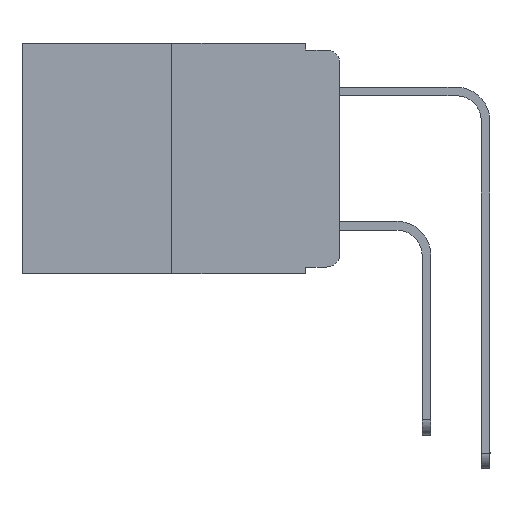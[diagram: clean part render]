
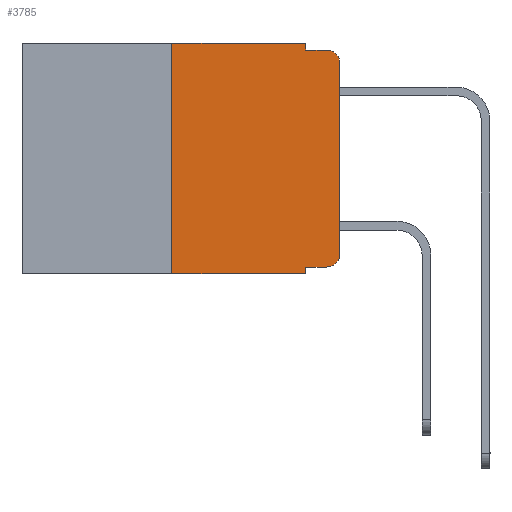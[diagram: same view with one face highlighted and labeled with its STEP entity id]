
A CAD part, left-side view. The second image highlights one B-rep face of the part: STEP entity #3785.
In plain terms, the highlighted planar face has unit normal (-1, 0, 0).
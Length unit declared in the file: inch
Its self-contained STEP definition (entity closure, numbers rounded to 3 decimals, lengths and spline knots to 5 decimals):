
#272 = LINE ( 'NONE', #19175, #15373 ) ;
#403 = CARTESIAN_POINT ( 'NONE',  ( 0., 0.25, 0. ) ) ;
#550 = VECTOR ( 'NONE', #16268, 39.37008 ) ;
#668 = VERTEX_POINT ( 'NONE', #17638 ) ;
#694 = CARTESIAN_POINT ( 'NONE',  ( 0., 0.051, -0.01 ) ) ;
#1282 = DIRECTION ( 'NONE',  ( 0., -1., 0. ) ) ;
#1435 = ORIENTED_EDGE ( 'NONE', *, *, #10564, .T. ) ;
#1475 = VERTEX_POINT ( 'NONE', #15623 ) ;
#1522 = DIRECTION ( 'NONE',  ( 0., -1., 0. ) ) ;
#1598 = CARTESIAN_POINT ( 'NONE',  ( 0., 0.02, -0.03 ) ) ;
#1801 = ORIENTED_EDGE ( 'NONE', *, *, #5862, .F. ) ;
#2607 = EDGE_CURVE ( 'NONE', #5838, #4358, #6332, .T. ) ;
#2641 = VERTEX_POINT ( 'NONE', #694 ) ;
#2734 = DIRECTION ( 'NONE',  ( 1., 0., 0. ) ) ;
#2908 = CIRCLE ( 'NONE', #12772, 0.02 ) ;
#3041 = ORIENTED_EDGE ( 'NONE', *, *, #8860, .F. ) ;
#3785 = ADVANCED_FACE ( 'NONE', ( #19972 ), #5840, .F. ) ;
#4199 = EDGE_CURVE ( 'NONE', #2641, #15779, #15564, .T. ) ;
#4358 = VERTEX_POINT ( 'NONE', #5074 ) ;
#4438 = VERTEX_POINT ( 'NONE', #11540 ) ;
#4927 = CIRCLE ( 'NONE', #16407, 0.02 ) ;
#5074 = CARTESIAN_POINT ( 'NONE',  ( 0., 0.051, 0. ) ) ;
#5301 = CARTESIAN_POINT ( 'NONE',  ( 0., 0.051, 0. ) ) ;
#5365 = LINE ( 'NONE', #9783, #550 ) ;
#5838 = VERTEX_POINT ( 'NONE', #15983 ) ;
#5839 = VERTEX_POINT ( 'NONE', #11443 ) ;
#5840 = PLANE ( 'NONE',  #17821 ) ;
#5862 = EDGE_CURVE ( 'NONE', #20322, #5838, #8253, .T. ) ;
#6332 = LINE ( 'NONE', #6436, #11780 ) ;
#6436 = CARTESIAN_POINT ( 'NONE',  ( 0., 0.473, 0. ) ) ;
#6742 = DIRECTION ( 'NONE',  ( -1., 0., 0. ) ) ;
#7667 = EDGE_LOOP ( 'NONE', ( #11766, #1435, #14814, #20324, #12751, #1801, #14634, #3041, #14861, #11894 ) ) ;
#7842 = DIRECTION ( 'NONE',  ( 0., -1., 0. ) ) ;
#8253 = LINE ( 'NONE', #403, #8597 ) ;
#8597 = VECTOR ( 'NONE', #11545, 39.37008 ) ;
#8860 = EDGE_CURVE ( 'NONE', #1475, #4438, #19435, .T. ) ;
#9343 = CARTESIAN_POINT ( 'NONE',  ( 0., 0.473, -0.343 ) ) ;
#9572 = CARTESIAN_POINT ( 'NONE',  ( 0., 0.25, -0.343 ) ) ;
#9783 = CARTESIAN_POINT ( 'NONE',  ( 0., 0., 0. ) ) ;
#10564 = EDGE_CURVE ( 'NONE', #668, #15779, #2908, .T. ) ;
#10661 = EDGE_CURVE ( 'NONE', #18608, #5839, #4927, .T. ) ;
#11046 = CARTESIAN_POINT ( 'NONE',  ( 0., 0.02, -0.01 ) ) ;
#11156 = VECTOR ( 'NONE', #14761, 39.37008 ) ;
#11443 = CARTESIAN_POINT ( 'NONE',  ( 0., 0., -0.313 ) ) ;
#11540 = CARTESIAN_POINT ( 'NONE',  ( 0., 0.051, -0.343 ) ) ;
#11545 = DIRECTION ( 'NONE',  ( 0., 0., 1. ) ) ;
#11766 = ORIENTED_EDGE ( 'NONE', *, *, #17537, .T. ) ;
#11780 = VECTOR ( 'NONE', #1282, 39.37008 ) ;
#11827 = EDGE_CURVE ( 'NONE', #20322, #4438, #12431, .T. ) ;
#11894 = ORIENTED_EDGE ( 'NONE', *, *, #10661, .T. ) ;
#12172 = CARTESIAN_POINT ( 'NONE',  ( 0., 0.051, -0.333 ) ) ;
#12431 = LINE ( 'NONE', #9343, #12601 ) ;
#12601 = VECTOR ( 'NONE', #1522, 39.37008 ) ;
#12751 = ORIENTED_EDGE ( 'NONE', *, *, #2607, .F. ) ;
#12772 = AXIS2_PLACEMENT_3D ( 'NONE', #1598, #6742, #14370 ) ;
#12940 = VECTOR ( 'NONE', #7842, 39.37008 ) ;
#13179 = CARTESIAN_POINT ( 'NONE',  ( 0., 0.02, -0.333 ) ) ;
#13204 = CARTESIAN_POINT ( 'NONE',  ( 0., 0.02, -0.313 ) ) ;
#13825 = DIRECTION ( 'NONE',  ( 0., -1., 0. ) ) ;
#14370 = DIRECTION ( 'NONE',  ( 0., 0., -1. ) ) ;
#14634 = ORIENTED_EDGE ( 'NONE', *, *, #11827, .T. ) ;
#14675 = DIRECTION ( 'NONE',  ( 0., 0., -1. ) ) ;
#14761 = DIRECTION ( 'NONE',  ( 0., 0., -1. ) ) ;
#14814 = ORIENTED_EDGE ( 'NONE', *, *, #4199, .F. ) ;
#14861 = ORIENTED_EDGE ( 'NONE', *, *, #19692, .T. ) ;
#15373 = VECTOR ( 'NONE', #17812, 39.37008 ) ;
#15564 = LINE ( 'NONE', #18573, #12940 ) ;
#15623 = CARTESIAN_POINT ( 'NONE',  ( 0., 0.051, -0.333 ) ) ;
#15671 = LINE ( 'NONE', #12172, #16097 ) ;
#15779 = VERTEX_POINT ( 'NONE', #11046 ) ;
#15983 = CARTESIAN_POINT ( 'NONE',  ( 0., 0.25, 0. ) ) ;
#16097 = VECTOR ( 'NONE', #13825, 39.37008 ) ;
#16268 = DIRECTION ( 'NONE',  ( 0., 0., 1. ) ) ;
#16407 = AXIS2_PLACEMENT_3D ( 'NONE', #13204, #17874, #14675 ) ;
#16843 = CARTESIAN_POINT ( 'NONE',  ( 0., 0.473, 0. ) ) ;
#17351 = DIRECTION ( 'NONE',  ( 0., 0., -1. ) ) ;
#17537 = EDGE_CURVE ( 'NONE', #5839, #668, #5365, .T. ) ;
#17638 = CARTESIAN_POINT ( 'NONE',  ( 0., 0., -0.03 ) ) ;
#17812 = DIRECTION ( 'NONE',  ( 0., 0., -1. ) ) ;
#17821 = AXIS2_PLACEMENT_3D ( 'NONE', #16843, #2734, #17351 ) ;
#17874 = DIRECTION ( 'NONE',  ( -1., 0., 0. ) ) ;
#17987 = EDGE_CURVE ( 'NONE', #4358, #2641, #272, .T. ) ;
#18573 = CARTESIAN_POINT ( 'NONE',  ( 0., 0.051, -0.01 ) ) ;
#18608 = VERTEX_POINT ( 'NONE', #13179 ) ;
#19175 = CARTESIAN_POINT ( 'NONE',  ( 0., 0.051, 0. ) ) ;
#19435 = LINE ( 'NONE', #5301, #11156 ) ;
#19692 = EDGE_CURVE ( 'NONE', #1475, #18608, #15671, .T. ) ;
#19972 = FACE_OUTER_BOUND ( 'NONE', #7667, .T. ) ;
#20322 = VERTEX_POINT ( 'NONE', #9572 ) ;
#20324 = ORIENTED_EDGE ( 'NONE', *, *, #17987, .F. ) ;
